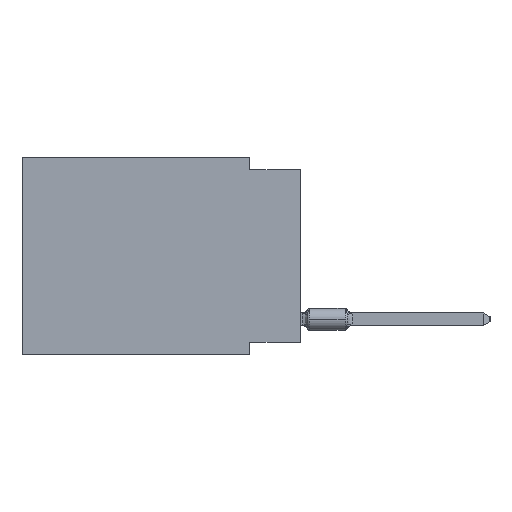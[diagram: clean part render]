
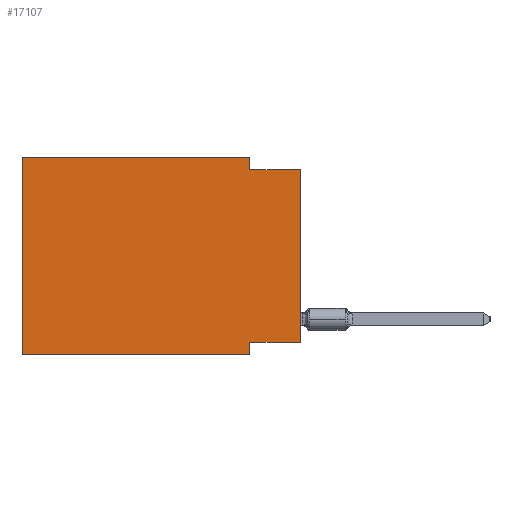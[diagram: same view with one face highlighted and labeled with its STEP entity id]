
A CAD part, left-side view. The second image highlights one B-rep face of the part: STEP entity #17107.
In plain terms, the highlighted planar face has unit normal (-1, 0, 0).
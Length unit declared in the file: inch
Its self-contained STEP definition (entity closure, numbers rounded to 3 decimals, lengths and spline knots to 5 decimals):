
#1068 = CARTESIAN_POINT ( 'NONE',  ( 0., 0.1, 0. ) ) ;
#2381 = VECTOR ( 'NONE', #8501, 39.37008 ) ;
#2448 = EDGE_CURVE ( 'NONE', #17995, #38090, #31705, .T. ) ;
#2509 = EDGE_CURVE ( 'NONE', #23768, #16121, #11743, .T. ) ;
#2844 = LINE ( 'NONE', #11973, #30830 ) ;
#2984 = CARTESIAN_POINT ( 'NONE',  ( 0., 0.55, 0. ) ) ;
#3595 = CARTESIAN_POINT ( 'NONE',  ( 0., 0., -0.025 ) ) ;
#3804 = LINE ( 'NONE', #3595, #18608 ) ;
#3881 = ORIENTED_EDGE ( 'NONE', *, *, #33532, .F. ) ;
#4745 = DIRECTION ( 'NONE',  ( 0., 0., -1. ) ) ;
#4792 = ORIENTED_EDGE ( 'NONE', *, *, #42453, .T. ) ;
#5600 = CARTESIAN_POINT ( 'NONE',  ( 0., 0., -0.365 ) ) ;
#6874 = VECTOR ( 'NONE', #4745, 39.37008 ) ;
#7662 = EDGE_LOOP ( 'NONE', ( #38521, #8468, #8002, #21697, #28586, #4792, #3881, #16325 ) ) ;
#8002 = ORIENTED_EDGE ( 'NONE', *, *, #39691, .F. ) ;
#8197 = DIRECTION ( 'NONE',  ( 0., 0., -1. ) ) ;
#8468 = ORIENTED_EDGE ( 'NONE', *, *, #12068, .F. ) ;
#8501 = DIRECTION ( 'NONE',  ( 0., 0., 1. ) ) ;
#11641 = CARTESIAN_POINT ( 'NONE',  ( 0., 0., -0.365 ) ) ;
#11743 = LINE ( 'NONE', #38231, #2381 ) ;
#11973 = CARTESIAN_POINT ( 'NONE',  ( 0., 0.55, -0.39 ) ) ;
#12068 = EDGE_CURVE ( 'NONE', #38255, #16121, #3804, .T. ) ;
#12767 = DIRECTION ( 'NONE',  ( 0., 0., 1. ) ) ;
#14124 = AXIS2_PLACEMENT_3D ( 'NONE', #35122, #27952, #18623 ) ;
#15016 = CARTESIAN_POINT ( 'NONE',  ( 0., 0.55, 0. ) ) ;
#16121 = VERTEX_POINT ( 'NONE', #40505 ) ;
#16325 = ORIENTED_EDGE ( 'NONE', *, *, #23511, .F. ) ;
#17107 = ADVANCED_FACE ( 'NONE', ( #41422 ), #38165, .F. ) ;
#17995 = VERTEX_POINT ( 'NONE', #26887 ) ;
#18603 = LINE ( 'NONE', #24266, #41787 ) ;
#18608 = VECTOR ( 'NONE', #27247, 39.37008 ) ;
#18623 = DIRECTION ( 'NONE',  ( 0., 0., -1. ) ) ;
#19001 = VECTOR ( 'NONE', #38017, 39.37008 ) ;
#21462 = CARTESIAN_POINT ( 'NONE',  ( 0., 0.1, -0.39 ) ) ;
#21625 = VECTOR ( 'NONE', #12767, 39.37008 ) ;
#21697 = ORIENTED_EDGE ( 'NONE', *, *, #2448, .F. ) ;
#22966 = VERTEX_POINT ( 'NONE', #38435 ) ;
#23511 = EDGE_CURVE ( 'NONE', #23768, #22966, #35560, .T. ) ;
#23768 = VERTEX_POINT ( 'NONE', #11641 ) ;
#24266 = CARTESIAN_POINT ( 'NONE',  ( 0., 0.1, 0. ) ) ;
#24496 = LINE ( 'NONE', #21462, #6874 ) ;
#25214 = DIRECTION ( 'NONE',  ( 0., -1., 0. ) ) ;
#26887 = CARTESIAN_POINT ( 'NONE',  ( 0., 0.55, 0. ) ) ;
#27247 = DIRECTION ( 'NONE',  ( 0., -1., 0. ) ) ;
#27952 = DIRECTION ( 'NONE',  ( 1., 0., 0. ) ) ;
#28172 = CARTESIAN_POINT ( 'NONE',  ( 0., 0.1, -0.39 ) ) ;
#28586 = ORIENTED_EDGE ( 'NONE', *, *, #38139, .F. ) ;
#28612 = LINE ( 'NONE', #2984, #21625 ) ;
#30830 = VECTOR ( 'NONE', #25214, 39.37008 ) ;
#30912 = VERTEX_POINT ( 'NONE', #28172 ) ;
#31705 = LINE ( 'NONE', #15016, #19001 ) ;
#32288 = DIRECTION ( 'NONE',  ( 0., 1., 0. ) ) ;
#33532 = EDGE_CURVE ( 'NONE', #22966, #30912, #24496, .T. ) ;
#35122 = CARTESIAN_POINT ( 'NONE',  ( 0., 0.55, 0. ) ) ;
#35560 = LINE ( 'NONE', #5600, #37297 ) ;
#37283 = CARTESIAN_POINT ( 'NONE',  ( 0., 0.1, -0.025 ) ) ;
#37297 = VECTOR ( 'NONE', #32288, 39.37008 ) ;
#38017 = DIRECTION ( 'NONE',  ( 0., -1., 0. ) ) ;
#38090 = VERTEX_POINT ( 'NONE', #1068 ) ;
#38139 = EDGE_CURVE ( 'NONE', #40695, #17995, #28612, .T. ) ;
#38165 = PLANE ( 'NONE',  #14124 ) ;
#38231 = CARTESIAN_POINT ( 'NONE',  ( 0., 0., 0. ) ) ;
#38255 = VERTEX_POINT ( 'NONE', #37283 ) ;
#38435 = CARTESIAN_POINT ( 'NONE',  ( 0., 0.1, -0.365 ) ) ;
#38521 = ORIENTED_EDGE ( 'NONE', *, *, #2509, .T. ) ;
#39691 = EDGE_CURVE ( 'NONE', #38090, #38255, #18603, .T. ) ;
#40048 = CARTESIAN_POINT ( 'NONE',  ( 0., 0.55, -0.39 ) ) ;
#40505 = CARTESIAN_POINT ( 'NONE',  ( 0., 0., -0.025 ) ) ;
#40695 = VERTEX_POINT ( 'NONE', #40048 ) ;
#41422 = FACE_OUTER_BOUND ( 'NONE', #7662, .T. ) ;
#41787 = VECTOR ( 'NONE', #8197, 39.37008 ) ;
#42453 = EDGE_CURVE ( 'NONE', #40695, #30912, #2844, .T. ) ;
